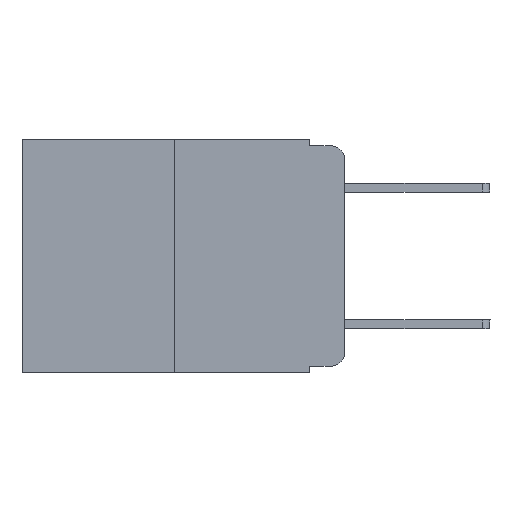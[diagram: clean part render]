
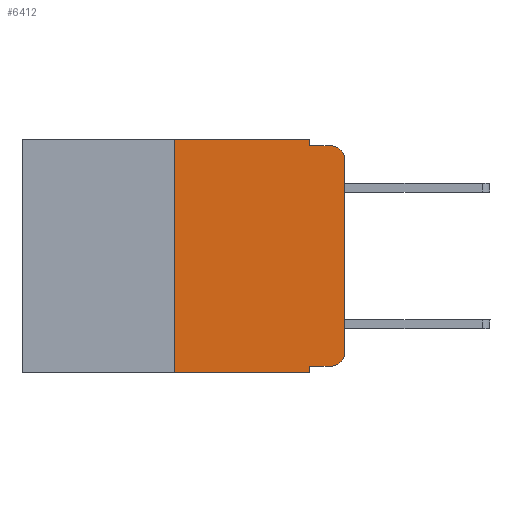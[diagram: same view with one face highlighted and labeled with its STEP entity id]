
A CAD part, left-side view. The second image highlights one B-rep face of the part: STEP entity #6412.
In plain terms, the highlighted planar face has unit normal (-1, 0, 0).
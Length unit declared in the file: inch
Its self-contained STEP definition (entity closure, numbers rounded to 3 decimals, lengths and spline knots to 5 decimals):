
#59 = EDGE_CURVE ( 'NONE', #8349, #3850, #5780, .T. ) ;
#453 = VERTEX_POINT ( 'NONE', #7095 ) ;
#728 = ORIENTED_EDGE ( 'NONE', *, *, #12448, .T. ) ;
#747 = VERTEX_POINT ( 'NONE', #7367 ) ;
#1410 = ORIENTED_EDGE ( 'NONE', *, *, #7693, .F. ) ;
#1603 = CARTESIAN_POINT ( 'NONE',  ( 0., 0.473, -0.343 ) ) ;
#1609 = EDGE_CURVE ( 'NONE', #3850, #453, #14421, .T. ) ;
#1964 = CARTESIAN_POINT ( 'NONE',  ( 0., 0.051, -0.333 ) ) ;
#2177 = DIRECTION ( 'NONE',  ( 0., 0., -1. ) ) ;
#2376 = CIRCLE ( 'NONE', #11212, 0.02 ) ;
#2388 = CARTESIAN_POINT ( 'NONE',  ( 0., 0.02, -0.03 ) ) ;
#2507 = CARTESIAN_POINT ( 'NONE',  ( 0., 0., 0. ) ) ;
#2582 = DIRECTION ( 'NONE',  ( 0., -1., 0. ) ) ;
#2602 = LINE ( 'NONE', #1964, #2957 ) ;
#2664 = FACE_OUTER_BOUND ( 'NONE', #14288, .T. ) ;
#2957 = VECTOR ( 'NONE', #3281, 39.37008 ) ;
#2988 = CARTESIAN_POINT ( 'NONE',  ( 0., 0.25, 0. ) ) ;
#3112 = VERTEX_POINT ( 'NONE', #8569 ) ;
#3281 = DIRECTION ( 'NONE',  ( 0., -1., 0. ) ) ;
#3284 = CARTESIAN_POINT ( 'NONE',  ( 0., 0.473, 0. ) ) ;
#3850 = VERTEX_POINT ( 'NONE', #12542 ) ;
#4013 = CARTESIAN_POINT ( 'NONE',  ( 0., 0.051, 0. ) ) ;
#4029 = CARTESIAN_POINT ( 'NONE',  ( 0., 0.051, -0.01 ) ) ;
#5320 = CARTESIAN_POINT ( 'NONE',  ( 0., 0.25, -0.343 ) ) ;
#5615 = CARTESIAN_POINT ( 'NONE',  ( 0., 0.473, 0. ) ) ;
#5780 = LINE ( 'NONE', #2507, #8910 ) ;
#5792 = VECTOR ( 'NONE', #7103, 39.37008 ) ;
#5834 = DIRECTION ( 'NONE',  ( 1., 0., 0. ) ) ;
#6021 = ORIENTED_EDGE ( 'NONE', *, *, #15929, .T. ) ;
#6218 = DIRECTION ( 'NONE',  ( 0., 0., -1. ) ) ;
#6412 = ADVANCED_FACE ( 'NONE', ( #2664 ), #13170, .F. ) ;
#6553 = ORIENTED_EDGE ( 'NONE', *, *, #59, .T. ) ;
#7044 = AXIS2_PLACEMENT_3D ( 'NONE', #2388, #9858, #2177 ) ;
#7095 = CARTESIAN_POINT ( 'NONE',  ( 0., 0.02, -0.01 ) ) ;
#7103 = DIRECTION ( 'NONE',  ( 0., -1., 0. ) ) ;
#7195 = CARTESIAN_POINT ( 'NONE',  ( 0., 0.25, 0. ) ) ;
#7352 = VERTEX_POINT ( 'NONE', #7778 ) ;
#7367 = CARTESIAN_POINT ( 'NONE',  ( 0., 0.051, -0.343 ) ) ;
#7559 = DIRECTION ( 'NONE',  ( 0., 0., -1. ) ) ;
#7693 = EDGE_CURVE ( 'NONE', #8322, #14942, #11921, .T. ) ;
#7778 = CARTESIAN_POINT ( 'NONE',  ( 0., 0.02, -0.333 ) ) ;
#8246 = EDGE_CURVE ( 'NONE', #14967, #8322, #12494, .T. ) ;
#8322 = VERTEX_POINT ( 'NONE', #7195 ) ;
#8349 = VERTEX_POINT ( 'NONE', #9666 ) ;
#8569 = CARTESIAN_POINT ( 'NONE',  ( 0., 0.051, -0.333 ) ) ;
#8607 = LINE ( 'NONE', #13600, #13166 ) ;
#8676 = CARTESIAN_POINT ( 'NONE',  ( 0., 0.051, -0.01 ) ) ;
#8711 = VECTOR ( 'NONE', #11818, 39.37008 ) ;
#8910 = VECTOR ( 'NONE', #12594, 39.37008 ) ;
#9066 = ORIENTED_EDGE ( 'NONE', *, *, #8246, .F. ) ;
#9089 = AXIS2_PLACEMENT_3D ( 'NONE', #5615, #5834, #14430 ) ;
#9666 = CARTESIAN_POINT ( 'NONE',  ( 0., 0., -0.313 ) ) ;
#9858 = DIRECTION ( 'NONE',  ( -1., 0., 0. ) ) ;
#10341 = VECTOR ( 'NONE', #12898, 39.37008 ) ;
#10438 = VECTOR ( 'NONE', #2582, 39.37008 ) ;
#10624 = EDGE_CURVE ( 'NONE', #3112, #7352, #2602, .T. ) ;
#10658 = LINE ( 'NONE', #4029, #10438 ) ;
#11010 = VECTOR ( 'NONE', #7559, 39.37008 ) ;
#11212 = AXIS2_PLACEMENT_3D ( 'NONE', #12791, #11475, #14149 ) ;
#11397 = EDGE_CURVE ( 'NONE', #3112, #747, #8607, .T. ) ;
#11475 = DIRECTION ( 'NONE',  ( -1., 0., 0. ) ) ;
#11593 = LINE ( 'NONE', #14994, #11010 ) ;
#11818 = DIRECTION ( 'NONE',  ( 0., 0., 1. ) ) ;
#11921 = LINE ( 'NONE', #3284, #5792 ) ;
#11948 = ORIENTED_EDGE ( 'NONE', *, *, #11397, .F. ) ;
#11954 = LINE ( 'NONE', #1603, #10341 ) ;
#12319 = VERTEX_POINT ( 'NONE', #8676 ) ;
#12446 = EDGE_CURVE ( 'NONE', #12319, #453, #10658, .T. ) ;
#12448 = EDGE_CURVE ( 'NONE', #7352, #8349, #2376, .T. ) ;
#12494 = LINE ( 'NONE', #2988, #8711 ) ;
#12542 = CARTESIAN_POINT ( 'NONE',  ( 0., 0., -0.03 ) ) ;
#12594 = DIRECTION ( 'NONE',  ( 0., 0., 1. ) ) ;
#12791 = CARTESIAN_POINT ( 'NONE',  ( 0., 0.02, -0.313 ) ) ;
#12898 = DIRECTION ( 'NONE',  ( 0., -1., 0. ) ) ;
#13166 = VECTOR ( 'NONE', #6218, 39.37008 ) ;
#13170 = PLANE ( 'NONE',  #9089 ) ;
#13600 = CARTESIAN_POINT ( 'NONE',  ( 0., 0.051, 0. ) ) ;
#13725 = ORIENTED_EDGE ( 'NONE', *, *, #1609, .T. ) ;
#13943 = ORIENTED_EDGE ( 'NONE', *, *, #12446, .F. ) ;
#14149 = DIRECTION ( 'NONE',  ( 0., 0., -1. ) ) ;
#14288 = EDGE_LOOP ( 'NONE', ( #6553, #13725, #13943, #15270, #1410, #9066, #6021, #11948, #14572, #728 ) ) ;
#14421 = CIRCLE ( 'NONE', #7044, 0.02 ) ;
#14430 = DIRECTION ( 'NONE',  ( 0., 0., -1. ) ) ;
#14572 = ORIENTED_EDGE ( 'NONE', *, *, #10624, .T. ) ;
#14790 = EDGE_CURVE ( 'NONE', #14942, #12319, #11593, .T. ) ;
#14942 = VERTEX_POINT ( 'NONE', #4013 ) ;
#14967 = VERTEX_POINT ( 'NONE', #5320 ) ;
#14994 = CARTESIAN_POINT ( 'NONE',  ( 0., 0.051, 0. ) ) ;
#15270 = ORIENTED_EDGE ( 'NONE', *, *, #14790, .F. ) ;
#15929 = EDGE_CURVE ( 'NONE', #14967, #747, #11954, .T. ) ;
